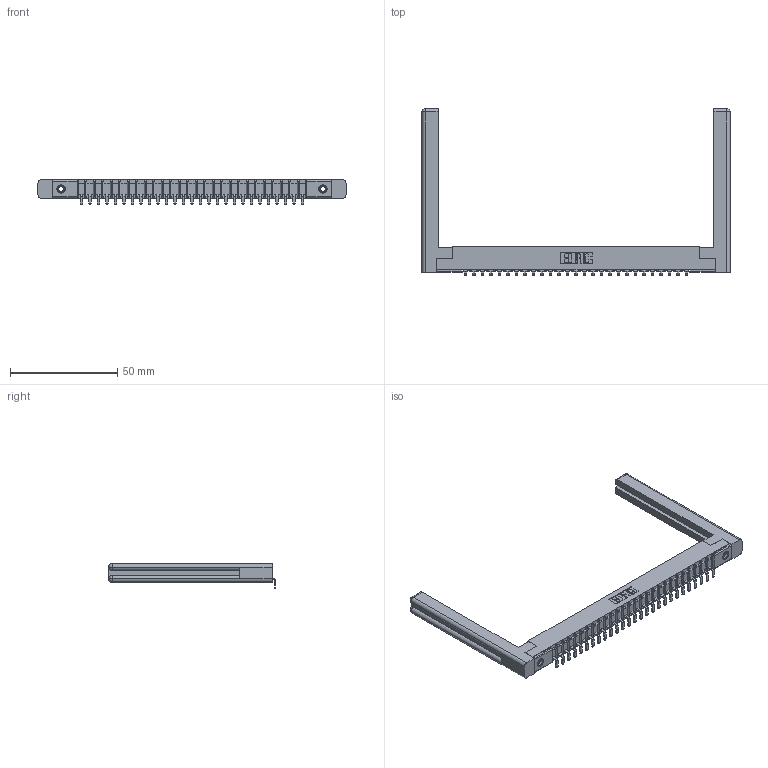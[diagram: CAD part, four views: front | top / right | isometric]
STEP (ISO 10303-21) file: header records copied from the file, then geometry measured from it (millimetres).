
FILE_DESCRIPTION (( 'STEP AP203' ), '1' );
FILE_NAME ('357-027-453-158.STEP', '2020-10-01T19:48:55', ( '' ), ( '' ), 'SwSTEP 2.0', 'SolidWorks 2020', '' );
FILE_SCHEMA (( 'CONFIG_CONTROL_DESIGN' ));
Length unit declared in the file: inch
Products named in the file (5): 307 Part_.156 Dia Mounting Holes; 307-290-002_553; 307-220-058; 357-027-453-158; 345-250-001_345-250-001-102
Assembly tree (32 placements, depth 2):
  357-027-453-158
    307 Part_.156 Dia Mounting Holes
    307-290-002_553  x27
    307-220-058  x2
    345-250-001_345-250-001-102  x2
Bounding box: 143.61 x 77.64 x 11.51 mm (x, y, z)
Volume: 17161.8 mm3; surface area: 22559.3 mm2
Topology: 32 solids, 32 shells, 2394 faces, 7265 edges, 4754 vertices
Faces by surface type: plane 1423, cylinder 891, sphere 56, torus 12, cone 12
Entity records: 28483 total; most frequent: CARTESIAN_POINT 4811, ORIENTED_EDGE 4740, DIRECTION 4642, EDGE_CURVE 2370, LINE 1804, VECTOR 1804, VERTEX_POINT 1534, AXIS2_PLACEMENT_3D 1419
